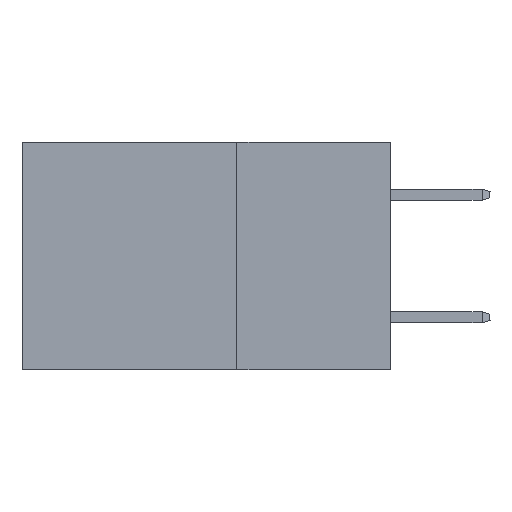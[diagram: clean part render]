
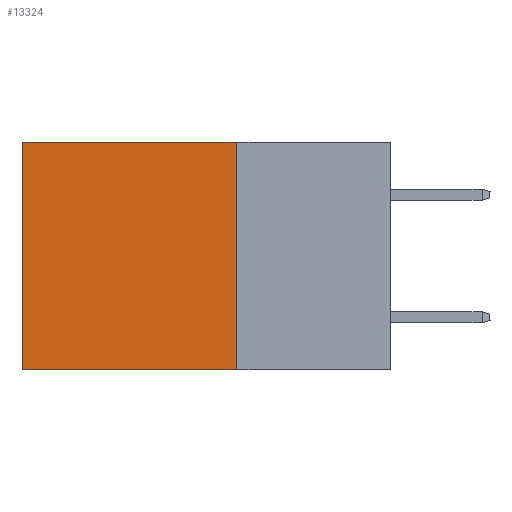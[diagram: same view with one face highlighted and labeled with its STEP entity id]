
A CAD part, left-side view. The second image highlights one B-rep face of the part: STEP entity #13324.
In plain terms, the highlighted planar face has unit normal (-1, 0, 0).
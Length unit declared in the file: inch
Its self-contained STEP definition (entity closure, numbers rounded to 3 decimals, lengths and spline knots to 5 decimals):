
#343 = ORIENTED_EDGE ( 'NONE', *, *, #9711, .T. ) ;
#1190 = CARTESIAN_POINT ( 'NONE',  ( 0.2875, 0.25, -0.37 ) ) ;
#1633 = ORIENTED_EDGE ( 'NONE', *, *, #12711, .T. ) ;
#2433 = VECTOR ( 'NONE', #3254, 39.37008 ) ;
#3147 = CARTESIAN_POINT ( 'NONE',  ( 0.2875, 0.25, 0. ) ) ;
#3254 = DIRECTION ( 'NONE',  ( 0., 1., 0. ) ) ;
#3286 = CARTESIAN_POINT ( 'NONE',  ( 0.2875, 0.25, -0.37 ) ) ;
#4049 = DIRECTION ( 'NONE',  ( 0., 0., -1. ) ) ;
#4377 = CARTESIAN_POINT ( 'NONE',  ( 0.2875, 0.6, -0.37 ) ) ;
#5926 = ORIENTED_EDGE ( 'NONE', *, *, #13245, .F. ) ;
#6099 = VERTEX_POINT ( 'NONE', #3286 ) ;
#6547 = CARTESIAN_POINT ( 'NONE',  ( 0.2875, 0.6, 0. ) ) ;
#7201 = CARTESIAN_POINT ( 'NONE',  ( 0.2875, 0.25, 0. ) ) ;
#8062 = VERTEX_POINT ( 'NONE', #4377 ) ;
#8243 = AXIS2_PLACEMENT_3D ( 'NONE', #3147, #16360, #20054 ) ;
#9334 = VECTOR ( 'NONE', #4049, 39.37008 ) ;
#9711 = EDGE_CURVE ( 'NONE', #10963, #8062, #11477, .T. ) ;
#9918 = LINE ( 'NONE', #13184, #9334 ) ;
#10144 = FACE_OUTER_BOUND ( 'NONE', #10518, .T. ) ;
#10518 = EDGE_LOOP ( 'NONE', ( #343, #5926, #16300, #1633 ) ) ;
#10963 = VERTEX_POINT ( 'NONE', #6547 ) ;
#11477 = LINE ( 'NONE', #12355, #23571 ) ;
#12355 = CARTESIAN_POINT ( 'NONE',  ( 0.2875, 0.6, 0. ) ) ;
#12711 = EDGE_CURVE ( 'NONE', #23025, #10963, #23136, .T. ) ;
#13184 = CARTESIAN_POINT ( 'NONE',  ( 0.2875, 0.25, 0. ) ) ;
#13245 = EDGE_CURVE ( 'NONE', #6099, #8062, #18684, .T. ) ;
#13324 = ADVANCED_FACE ( 'NONE', ( #10144 ), #22021, .F. ) ;
#15960 = CARTESIAN_POINT ( 'NONE',  ( 0.2875, 0.25, 0. ) ) ;
#16300 = ORIENTED_EDGE ( 'NONE', *, *, #20851, .F. ) ;
#16360 = DIRECTION ( 'NONE',  ( 1., 0., 0. ) ) ;
#16609 = VECTOR ( 'NONE', #22247, 39.37008 ) ;
#18684 = LINE ( 'NONE', #1190, #2433 ) ;
#19563 = DIRECTION ( 'NONE',  ( 0., 0., -1. ) ) ;
#20054 = DIRECTION ( 'NONE',  ( 0., 0., -1. ) ) ;
#20851 = EDGE_CURVE ( 'NONE', #23025, #6099, #9918, .T. ) ;
#22021 = PLANE ( 'NONE',  #8243 ) ;
#22247 = DIRECTION ( 'NONE',  ( 0., 1., 0. ) ) ;
#23025 = VERTEX_POINT ( 'NONE', #15960 ) ;
#23136 = LINE ( 'NONE', #7201, #16609 ) ;
#23571 = VECTOR ( 'NONE', #19563, 39.37008 ) ;
